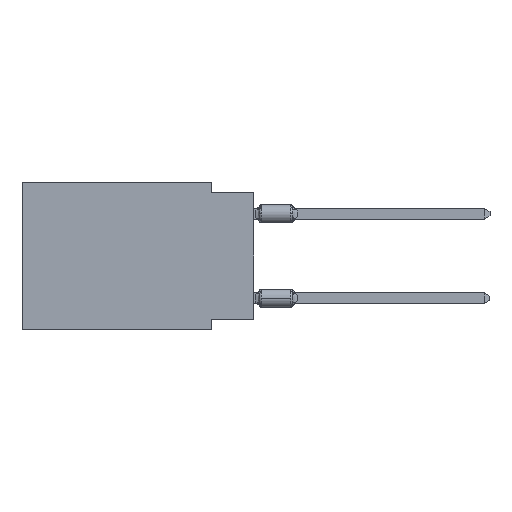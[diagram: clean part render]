
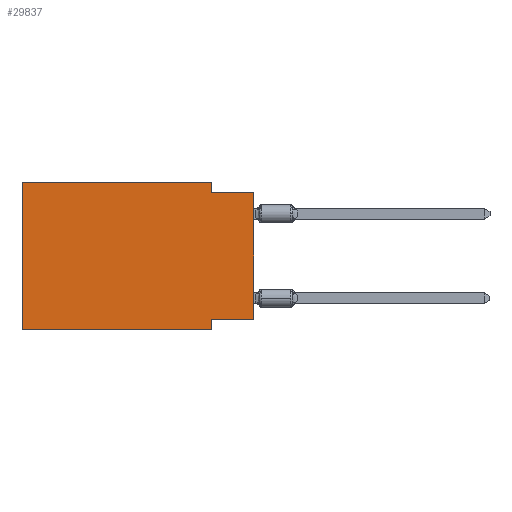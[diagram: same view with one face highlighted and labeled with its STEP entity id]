
A CAD part, left-side view. The second image highlights one B-rep face of the part: STEP entity #29837.
In plain terms, the highlighted planar face has unit normal (-1, 0, 0).
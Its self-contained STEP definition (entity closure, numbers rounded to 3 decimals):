
#189 = CARTESIAN_POINT ( 'NONE',  ( 0., 2.54, -8.255 ) ) ;
#1037 = LINE ( 'NONE', #1355, #11674 ) ;
#1355 = CARTESIAN_POINT ( 'NONE',  ( 0., 0., -8.255 ) ) ;
#2999 = CARTESIAN_POINT ( 'NONE',  ( 0., 13.97, -8.89 ) ) ;
#4168 = VECTOR ( 'NONE', #31178, 1000. ) ;
#4254 = CARTESIAN_POINT ( 'NONE',  ( 0., 0., 0. ) ) ;
#4614 = CARTESIAN_POINT ( 'NONE',  ( 0., 0., -0.635 ) ) ;
#4680 = EDGE_CURVE ( 'NONE', #6241, #22655, #21617, .T. ) ;
#5068 = CARTESIAN_POINT ( 'NONE',  ( 0., 13.97, 0. ) ) ;
#5804 = CARTESIAN_POINT ( 'NONE',  ( 0., 2.54, -8.89 ) ) ;
#5891 = ORIENTED_EDGE ( 'NONE', *, *, #4680, .F. ) ;
#6214 = ORIENTED_EDGE ( 'NONE', *, *, #19641, .F. ) ;
#6241 = VERTEX_POINT ( 'NONE', #15632 ) ;
#6728 = LINE ( 'NONE', #4614, #4168 ) ;
#7161 = VECTOR ( 'NONE', #11247, 1000. ) ;
#7509 = EDGE_CURVE ( 'NONE', #14784, #25778, #31872, .T. ) ;
#7643 = VERTEX_POINT ( 'NONE', #12761 ) ;
#8630 = VERTEX_POINT ( 'NONE', #13460 ) ;
#9114 = CARTESIAN_POINT ( 'NONE',  ( 0., 13.97, 0. ) ) ;
#9432 = CARTESIAN_POINT ( 'NONE',  ( 0., 2.54, -0.635 ) ) ;
#9476 = EDGE_CURVE ( 'NONE', #22655, #8630, #6728, .T. ) ;
#9700 = CARTESIAN_POINT ( 'NONE',  ( 0., 13.97, 0. ) ) ;
#11247 = DIRECTION ( 'NONE',  ( 0., -1., 0. ) ) ;
#11674 = VECTOR ( 'NONE', #15940, 1000. ) ;
#12551 = EDGE_LOOP ( 'NONE', ( #27366, #16910, #5891, #6214, #14074, #30015, #21073, #23401 ) ) ;
#12761 = CARTESIAN_POINT ( 'NONE',  ( 0., 2.54, -8.89 ) ) ;
#13460 = CARTESIAN_POINT ( 'NONE',  ( 0., 0., -0.635 ) ) ;
#14074 = ORIENTED_EDGE ( 'NONE', *, *, #7509, .F. ) ;
#14784 = VERTEX_POINT ( 'NONE', #2999 ) ;
#15580 = EDGE_CURVE ( 'NONE', #20912, #7643, #15853, .T. ) ;
#15632 = CARTESIAN_POINT ( 'NONE',  ( 0., 2.54, 0. ) ) ;
#15853 = LINE ( 'NONE', #5804, #26140 ) ;
#15940 = DIRECTION ( 'NONE',  ( 0., 1., 0. ) ) ;
#16257 = LINE ( 'NONE', #9114, #25641 ) ;
#16910 = ORIENTED_EDGE ( 'NONE', *, *, #9476, .F. ) ;
#17334 = CARTESIAN_POINT ( 'NONE',  ( 0., 13.97, 0. ) ) ;
#18283 = CARTESIAN_POINT ( 'NONE',  ( 0., 0., -8.255 ) ) ;
#18699 = DIRECTION ( 'NONE',  ( 0., 0., 1. ) ) ;
#18997 = DIRECTION ( 'NONE',  ( 0., -1., 0. ) ) ;
#19543 = VECTOR ( 'NONE', #26620, 1000. ) ;
#19641 = EDGE_CURVE ( 'NONE', #25778, #6241, #16257, .T. ) ;
#20912 = VERTEX_POINT ( 'NONE', #189 ) ;
#21073 = ORIENTED_EDGE ( 'NONE', *, *, #15580, .F. ) ;
#21126 = CARTESIAN_POINT ( 'NONE',  ( 0., 13.97, -8.89 ) ) ;
#21286 = LINE ( 'NONE', #4254, #23133 ) ;
#21617 = LINE ( 'NONE', #29054, #19543 ) ;
#22047 = FACE_OUTER_BOUND ( 'NONE', #12551, .T. ) ;
#22366 = EDGE_CURVE ( 'NONE', #14784, #7643, #23558, .T. ) ;
#22367 = PLANE ( 'NONE',  #26623 ) ;
#22655 = VERTEX_POINT ( 'NONE', #9432 ) ;
#23133 = VECTOR ( 'NONE', #18699, 1000. ) ;
#23318 = VERTEX_POINT ( 'NONE', #18283 ) ;
#23401 = ORIENTED_EDGE ( 'NONE', *, *, #30645, .F. ) ;
#23558 = LINE ( 'NONE', #21126, #7161 ) ;
#23800 = DIRECTION ( 'NONE',  ( 0., 0., -1. ) ) ;
#25641 = VECTOR ( 'NONE', #18997, 1000. ) ;
#25778 = VERTEX_POINT ( 'NONE', #5068 ) ;
#26140 = VECTOR ( 'NONE', #23800, 1000. ) ;
#26620 = DIRECTION ( 'NONE',  ( 0., 0., -1. ) ) ;
#26623 = AXIS2_PLACEMENT_3D ( 'NONE', #17334, #27371, #27204 ) ;
#27204 = DIRECTION ( 'NONE',  ( 0., 0., -1. ) ) ;
#27366 = ORIENTED_EDGE ( 'NONE', *, *, #28087, .T. ) ;
#27371 = DIRECTION ( 'NONE',  ( 1., 0., 0. ) ) ;
#28087 = EDGE_CURVE ( 'NONE', #23318, #8630, #21286, .T. ) ;
#29054 = CARTESIAN_POINT ( 'NONE',  ( 0., 2.54, 0. ) ) ;
#29457 = DIRECTION ( 'NONE',  ( 0., 0., 1. ) ) ;
#29837 = ADVANCED_FACE ( 'NONE', ( #22047 ), #22367, .F. ) ;
#30015 = ORIENTED_EDGE ( 'NONE', *, *, #22366, .T. ) ;
#30645 = EDGE_CURVE ( 'NONE', #23318, #20912, #1037, .T. ) ;
#31178 = DIRECTION ( 'NONE',  ( 0., -1., 0. ) ) ;
#31872 = LINE ( 'NONE', #9700, #31994 ) ;
#31994 = VECTOR ( 'NONE', #29457, 1000. ) ;
